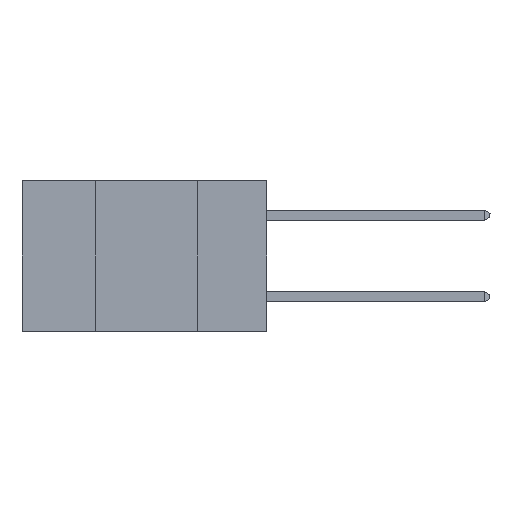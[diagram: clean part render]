
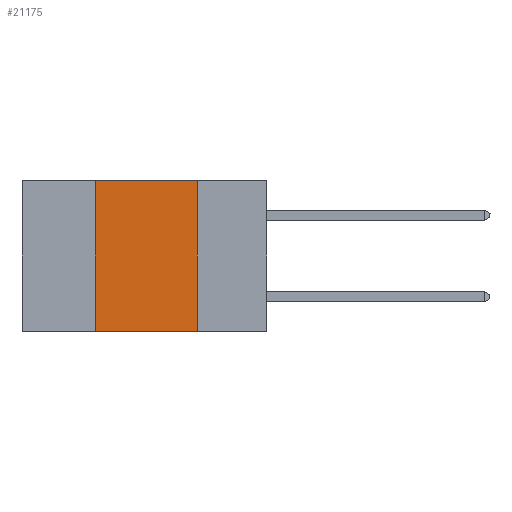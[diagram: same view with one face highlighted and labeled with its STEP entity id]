
A CAD part, left-side view. The second image highlights one B-rep face of the part: STEP entity #21175.
In plain terms, the highlighted planar face has unit normal (-1, 0, 0).
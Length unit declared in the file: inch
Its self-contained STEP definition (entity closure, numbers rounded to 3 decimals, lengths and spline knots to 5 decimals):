
#516 = CARTESIAN_POINT ( 'NONE',  ( 0., 0.42, 0. ) ) ;
#1587 = LINE ( 'NONE', #33004, #32607 ) ;
#5622 = CARTESIAN_POINT ( 'NONE',  ( 0., 0.17, 0. ) ) ;
#6190 = DIRECTION ( 'NONE',  ( 0., 0., -1. ) ) ;
#6827 = DIRECTION ( 'NONE',  ( 0., 0., -1. ) ) ;
#8197 = VERTEX_POINT ( 'NONE', #516 ) ;
#8314 = EDGE_CURVE ( 'NONE', #25714, #8197, #18547, .T. ) ;
#11312 = PLANE ( 'NONE',  #18756 ) ;
#11952 = DIRECTION ( 'NONE',  ( 0., 0., 1. ) ) ;
#12862 = VERTEX_POINT ( 'NONE', #23321 ) ;
#12893 = ORIENTED_EDGE ( 'NONE', *, *, #13967, .T. ) ;
#13967 = EDGE_CURVE ( 'NONE', #25714, #12862, #33560, .T. ) ;
#14615 = FACE_OUTER_BOUND ( 'NONE', #18658, .T. ) ;
#15366 = VECTOR ( 'NONE', #18843, 39.37008 ) ;
#16222 = CARTESIAN_POINT ( 'NONE',  ( 0., 0.6, 0. ) ) ;
#16690 = CARTESIAN_POINT ( 'NONE',  ( 0., 0.6, -0.37 ) ) ;
#16758 = CARTESIAN_POINT ( 'NONE',  ( 0., 0.6, 0. ) ) ;
#17350 = DIRECTION ( 'NONE',  ( 0., -1., 0. ) ) ;
#18547 = LINE ( 'NONE', #27429, #20587 ) ;
#18658 = EDGE_LOOP ( 'NONE', ( #25429, #30635, #23484, #12893 ) ) ;
#18756 = AXIS2_PLACEMENT_3D ( 'NONE', #16758, #29509, #6190 ) ;
#18843 = DIRECTION ( 'NONE',  ( 0., -1., 0. ) ) ;
#19908 = EDGE_CURVE ( 'NONE', #32060, #12862, #1587, .T. ) ;
#20587 = VECTOR ( 'NONE', #11952, 39.37008 ) ;
#21175 = ADVANCED_FACE ( 'NONE', ( #14615 ), #11312, .F. ) ;
#21819 = CARTESIAN_POINT ( 'NONE',  ( 0., 0.42, -0.37 ) ) ;
#23321 = CARTESIAN_POINT ( 'NONE',  ( 0., 0.17, -0.37 ) ) ;
#23484 = ORIENTED_EDGE ( 'NONE', *, *, #8314, .F. ) ;
#24181 = VECTOR ( 'NONE', #17350, 39.37008 ) ;
#25429 = ORIENTED_EDGE ( 'NONE', *, *, #19908, .F. ) ;
#25714 = VERTEX_POINT ( 'NONE', #21819 ) ;
#27429 = CARTESIAN_POINT ( 'NONE',  ( 0., 0.42, 0. ) ) ;
#28842 = LINE ( 'NONE', #16222, #15366 ) ;
#29509 = DIRECTION ( 'NONE',  ( 1., 0., 0. ) ) ;
#30635 = ORIENTED_EDGE ( 'NONE', *, *, #33012, .F. ) ;
#32060 = VERTEX_POINT ( 'NONE', #5622 ) ;
#32607 = VECTOR ( 'NONE', #6827, 39.37008 ) ;
#33004 = CARTESIAN_POINT ( 'NONE',  ( 0., 0.17, 0. ) ) ;
#33012 = EDGE_CURVE ( 'NONE', #8197, #32060, #28842, .T. ) ;
#33560 = LINE ( 'NONE', #16690, #24181 ) ;
